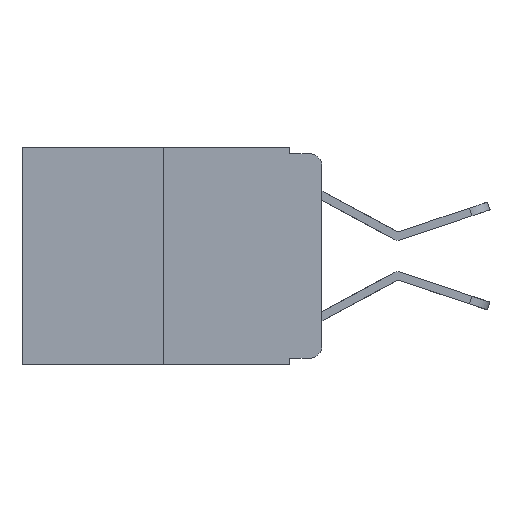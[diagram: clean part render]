
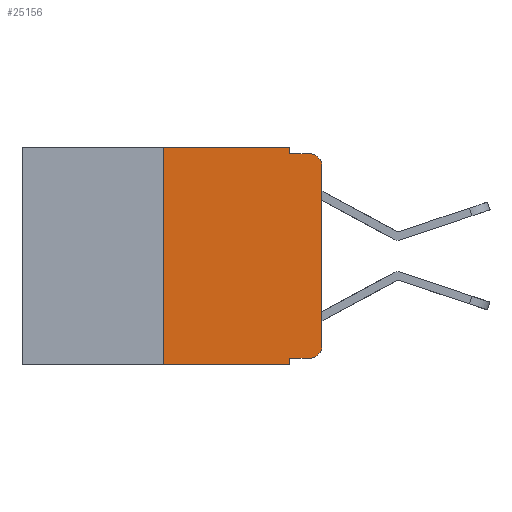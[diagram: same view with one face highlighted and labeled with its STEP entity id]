
A CAD part, left-side view. The second image highlights one B-rep face of the part: STEP entity #25156.
In plain terms, the highlighted planar face has unit normal (-1, 0, 0).
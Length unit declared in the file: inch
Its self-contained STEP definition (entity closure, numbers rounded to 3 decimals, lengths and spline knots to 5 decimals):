
#536 = VECTOR ( 'NONE', #5899, 39.37008 ) ;
#629 = AXIS2_PLACEMENT_3D ( 'NONE', #10456, #23962, #12459 ) ;
#724 = CARTESIAN_POINT ( 'NONE',  ( 0., 0.051, -0.343 ) ) ;
#730 = CARTESIAN_POINT ( 'NONE',  ( 0., 0.051, -0.333 ) ) ;
#1034 = EDGE_CURVE ( 'NONE', #17185, #9863, #14712, .T. ) ;
#1134 = EDGE_LOOP ( 'NONE', ( #9297, #7118, #10888, #4972, #19694, #16222, #17122, #20086, #24297, #17136 ) ) ;
#1166 = CARTESIAN_POINT ( 'NONE',  ( 0., 0.25, -0.343 ) ) ;
#1576 = CARTESIAN_POINT ( 'NONE',  ( 0., 0.051, 0. ) ) ;
#1806 = DIRECTION ( 'NONE',  ( 0., -1., 0. ) ) ;
#2873 = AXIS2_PLACEMENT_3D ( 'NONE', #19766, #8081, #21705 ) ;
#3980 = CARTESIAN_POINT ( 'NONE',  ( 0., 0., 0. ) ) ;
#4304 = CIRCLE ( 'NONE', #629, 0.02 ) ;
#4317 = LINE ( 'NONE', #13702, #16076 ) ;
#4856 = EDGE_CURVE ( 'NONE', #17118, #13207, #5824, .T. ) ;
#4972 = ORIENTED_EDGE ( 'NONE', *, *, #18186, .F. ) ;
#5047 = CARTESIAN_POINT ( 'NONE',  ( 0., 0.051, 0. ) ) ;
#5294 = DIRECTION ( 'NONE',  ( 0., -1., 0. ) ) ;
#5336 = CARTESIAN_POINT ( 'NONE',  ( 0., 0.051, -0.333 ) ) ;
#5824 = LINE ( 'NONE', #3980, #536 ) ;
#5899 = DIRECTION ( 'NONE',  ( 0., 0., 1. ) ) ;
#6353 = EDGE_CURVE ( 'NONE', #20114, #16834, #15054, .T. ) ;
#6748 = CARTESIAN_POINT ( 'NONE',  ( 0., 0., -0.313 ) ) ;
#7118 = ORIENTED_EDGE ( 'NONE', *, *, #18519, .T. ) ;
#7659 = VERTEX_POINT ( 'NONE', #14110 ) ;
#7828 = EDGE_CURVE ( 'NONE', #17185, #7659, #18273, .T. ) ;
#8066 = LINE ( 'NONE', #17102, #17877 ) ;
#8081 = DIRECTION ( 'NONE',  ( -1., 0., 0. ) ) ;
#8553 = CARTESIAN_POINT ( 'NONE',  ( 0., 0.473, 0. ) ) ;
#8650 = FACE_OUTER_BOUND ( 'NONE', #1134, .T. ) ;
#8723 = VERTEX_POINT ( 'NONE', #21008 ) ;
#9297 = ORIENTED_EDGE ( 'NONE', *, *, #4856, .T. ) ;
#9434 = VECTOR ( 'NONE', #21187, 39.37008 ) ;
#9611 = CARTESIAN_POINT ( 'NONE',  ( 0., 0.473, 0. ) ) ;
#9810 = CARTESIAN_POINT ( 'NONE',  ( 0., 0.25, 0. ) ) ;
#9863 = VERTEX_POINT ( 'NONE', #724 ) ;
#10456 = CARTESIAN_POINT ( 'NONE',  ( 0., 0.02, -0.313 ) ) ;
#10888 = ORIENTED_EDGE ( 'NONE', *, *, #23303, .F. ) ;
#11609 = CARTESIAN_POINT ( 'NONE',  ( 0., 0.051, -0.01 ) ) ;
#11997 = AXIS2_PLACEMENT_3D ( 'NONE', #8553, #24077, #12582 ) ;
#12296 = CARTESIAN_POINT ( 'NONE',  ( 0., 0.25, 0. ) ) ;
#12459 = DIRECTION ( 'NONE',  ( 0., 0., -1. ) ) ;
#12582 = DIRECTION ( 'NONE',  ( 0., 0., -1. ) ) ;
#13207 = VERTEX_POINT ( 'NONE', #23330 ) ;
#13702 = CARTESIAN_POINT ( 'NONE',  ( 0., 0.473, -0.343 ) ) ;
#13774 = VERTEX_POINT ( 'NONE', #11609 ) ;
#14110 = CARTESIAN_POINT ( 'NONE',  ( 0., 0.02, -0.333 ) ) ;
#14712 = LINE ( 'NONE', #1576, #9434 ) ;
#15054 = LINE ( 'NONE', #12296, #18923 ) ;
#15495 = LINE ( 'NONE', #9611, #21181 ) ;
#15922 = EDGE_CURVE ( 'NONE', #16834, #8723, #15495, .T. ) ;
#16076 = VECTOR ( 'NONE', #1806, 39.37008 ) ;
#16222 = ORIENTED_EDGE ( 'NONE', *, *, #6353, .F. ) ;
#16834 = VERTEX_POINT ( 'NONE', #9810 ) ;
#16869 = DIRECTION ( 'NONE',  ( 0., 0., -1. ) ) ;
#17102 = CARTESIAN_POINT ( 'NONE',  ( 0., 0.051, -0.01 ) ) ;
#17118 = VERTEX_POINT ( 'NONE', #6748 ) ;
#17122 = ORIENTED_EDGE ( 'NONE', *, *, #24902, .T. ) ;
#17136 = ORIENTED_EDGE ( 'NONE', *, *, #23934, .T. ) ;
#17185 = VERTEX_POINT ( 'NONE', #5336 ) ;
#17217 = LINE ( 'NONE', #5047, #22326 ) ;
#17877 = VECTOR ( 'NONE', #5294, 39.37008 ) ;
#18186 = EDGE_CURVE ( 'NONE', #8723, #13774, #17217, .T. ) ;
#18273 = LINE ( 'NONE', #730, #22745 ) ;
#18308 = DIRECTION ( 'NONE',  ( 0., -1., 0. ) ) ;
#18519 = EDGE_CURVE ( 'NONE', #13207, #21195, #20801, .T. ) ;
#18923 = VECTOR ( 'NONE', #23790, 39.37008 ) ;
#19694 = ORIENTED_EDGE ( 'NONE', *, *, #15922, .F. ) ;
#19766 = CARTESIAN_POINT ( 'NONE',  ( 0., 0.02, -0.03 ) ) ;
#20086 = ORIENTED_EDGE ( 'NONE', *, *, #1034, .F. ) ;
#20114 = VERTEX_POINT ( 'NONE', #1166 ) ;
#20201 = CARTESIAN_POINT ( 'NONE',  ( 0., 0.02, -0.01 ) ) ;
#20801 = CIRCLE ( 'NONE', #2873, 0.02 ) ;
#21008 = CARTESIAN_POINT ( 'NONE',  ( 0., 0.051, 0. ) ) ;
#21181 = VECTOR ( 'NONE', #23153, 39.37008 ) ;
#21187 = DIRECTION ( 'NONE',  ( 0., 0., -1. ) ) ;
#21195 = VERTEX_POINT ( 'NONE', #20201 ) ;
#21705 = DIRECTION ( 'NONE',  ( 0., 0., -1. ) ) ;
#22174 = PLANE ( 'NONE',  #11997 ) ;
#22326 = VECTOR ( 'NONE', #16869, 39.37008 ) ;
#22745 = VECTOR ( 'NONE', #18308, 39.37008 ) ;
#23153 = DIRECTION ( 'NONE',  ( 0., -1., 0. ) ) ;
#23303 = EDGE_CURVE ( 'NONE', #13774, #21195, #8066, .T. ) ;
#23330 = CARTESIAN_POINT ( 'NONE',  ( 0., 0., -0.03 ) ) ;
#23790 = DIRECTION ( 'NONE',  ( 0., 0., 1. ) ) ;
#23934 = EDGE_CURVE ( 'NONE', #7659, #17118, #4304, .T. ) ;
#23962 = DIRECTION ( 'NONE',  ( -1., 0., 0. ) ) ;
#24077 = DIRECTION ( 'NONE',  ( 1., 0., 0. ) ) ;
#24297 = ORIENTED_EDGE ( 'NONE', *, *, #7828, .T. ) ;
#24902 = EDGE_CURVE ( 'NONE', #20114, #9863, #4317, .T. ) ;
#25156 = ADVANCED_FACE ( 'NONE', ( #8650 ), #22174, .F. ) ;
